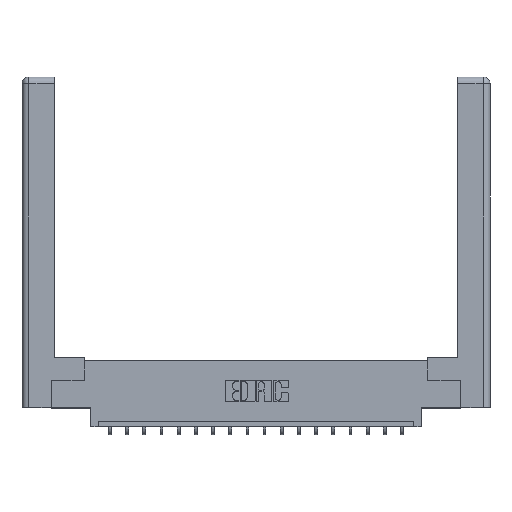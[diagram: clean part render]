
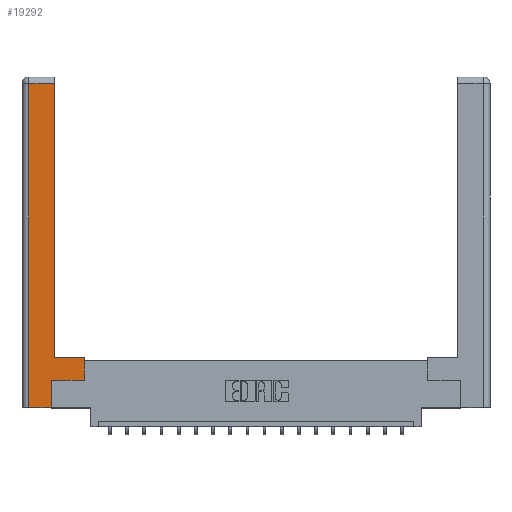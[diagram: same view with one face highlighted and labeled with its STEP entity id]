
A CAD part, top view. The second image highlights one B-rep face of the part: STEP entity #19292.
In plain terms, the highlighted planar face has unit normal (0, 0, 1).
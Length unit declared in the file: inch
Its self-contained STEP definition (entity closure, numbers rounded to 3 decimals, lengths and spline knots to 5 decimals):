
#159 = EDGE_CURVE ( 'NONE', #3786, #2519, #12593, .T. ) ;
#300 = EDGE_CURVE ( 'NONE', #6860, #7425, #4902, .T. ) ;
#514 = LINE ( 'NONE', #19225, #18014 ) ;
#951 = DIRECTION ( 'NONE',  ( -1., 0., 0. ) ) ;
#1025 = CARTESIAN_POINT ( 'NONE',  ( 0.565, 0.45, 0. ) ) ;
#1565 = CARTESIAN_POINT ( 'NONE',  ( 0.0615, 2.94, 0. ) ) ;
#1653 = ORIENTED_EDGE ( 'NONE', *, *, #16850, .T. ) ;
#1750 = ORIENTED_EDGE ( 'NONE', *, *, #300, .T. ) ;
#2519 = VERTEX_POINT ( 'NONE', #11934 ) ;
#2888 = DIRECTION ( 'NONE',  ( 0., 1., 0. ) ) ;
#2975 = DIRECTION ( 'NONE',  ( 1., 0., 0. ) ) ;
#3498 = CARTESIAN_POINT ( 'NONE',  ( 0.565, 0.245, 0. ) ) ;
#3678 = FACE_OUTER_BOUND ( 'NONE', #14730, .T. ) ;
#3786 = VERTEX_POINT ( 'NONE', #1025 ) ;
#3906 = CARTESIAN_POINT ( 'NONE',  ( 0., 0., 0. ) ) ;
#4070 = VERTEX_POINT ( 'NONE', #1565 ) ;
#4534 = CARTESIAN_POINT ( 'NONE',  ( 0.265, 0., 0. ) ) ;
#4902 = LINE ( 'NONE', #8746, #17951 ) ;
#5657 = DIRECTION ( 'NONE',  ( 0., 1., 0. ) ) ;
#5924 = ORIENTED_EDGE ( 'NONE', *, *, #6872, .T. ) ;
#6283 = LINE ( 'NONE', #10292, #14432 ) ;
#6556 = LINE ( 'NONE', #4534, #12621 ) ;
#6759 = ORIENTED_EDGE ( 'NONE', *, *, #8182, .T. ) ;
#6860 = VERTEX_POINT ( 'NONE', #7042 ) ;
#6872 = EDGE_CURVE ( 'NONE', #4070, #18617, #514, .T. ) ;
#7042 = CARTESIAN_POINT ( 'NONE',  ( 0.265, 0., 0. ) ) ;
#7152 = VECTOR ( 'NONE', #10842, 39.37008 ) ;
#7361 = DIRECTION ( 'NONE',  ( -1., 0., 0. ) ) ;
#7425 = VERTEX_POINT ( 'NONE', #11733 ) ;
#8073 = ORIENTED_EDGE ( 'NONE', *, *, #16611, .T. ) ;
#8082 = LINE ( 'NONE', #3498, #7152 ) ;
#8182 = EDGE_CURVE ( 'NONE', #19232, #4070, #11906, .T. ) ;
#8651 = VECTOR ( 'NONE', #11380, 39.37008 ) ;
#8746 = CARTESIAN_POINT ( 'NONE',  ( 0.265, 0.245, 0. ) ) ;
#10049 = EDGE_CURVE ( 'NONE', #2519, #19232, #15288, .T. ) ;
#10292 = CARTESIAN_POINT ( 'NONE',  ( 0.565, 0.45, 0. ) ) ;
#10531 = CARTESIAN_POINT ( 'NONE',  ( 0.0615, 2.94, 0. ) ) ;
#10842 = DIRECTION ( 'NONE',  ( 1., 0., 0. ) ) ;
#10862 = VECTOR ( 'NONE', #18126, 39.37008 ) ;
#10889 = ORIENTED_EDGE ( 'NONE', *, *, #10049, .T. ) ;
#11380 = DIRECTION ( 'NONE',  ( -1., 0., 0. ) ) ;
#11451 = DIRECTION ( 'NONE',  ( 0., 0., -1. ) ) ;
#11588 = EDGE_CURVE ( 'NONE', #7425, #14352, #8082, .T. ) ;
#11733 = CARTESIAN_POINT ( 'NONE',  ( 0.265, 0.245, 0. ) ) ;
#11906 = LINE ( 'NONE', #10531, #12377 ) ;
#11934 = CARTESIAN_POINT ( 'NONE',  ( 0.295, 0.45, 0. ) ) ;
#12377 = VECTOR ( 'NONE', #7361, 39.37008 ) ;
#12593 = LINE ( 'NONE', #18756, #8651 ) ;
#12621 = VECTOR ( 'NONE', #2975, 39.37008 ) ;
#13399 = ORIENTED_EDGE ( 'NONE', *, *, #159, .T. ) ;
#14352 = VERTEX_POINT ( 'NONE', #14885 ) ;
#14432 = VECTOR ( 'NONE', #2888, 39.37008 ) ;
#14730 = EDGE_LOOP ( 'NONE', ( #10889, #6759, #5924, #1653, #1750, #16818, #8073, #13399 ) ) ;
#14885 = CARTESIAN_POINT ( 'NONE',  ( 0.565, 0.245, 0. ) ) ;
#14909 = DIRECTION ( 'NONE',  ( 0., -1., 0. ) ) ;
#15288 = LINE ( 'NONE', #16642, #10862 ) ;
#16611 = EDGE_CURVE ( 'NONE', #14352, #3786, #6283, .T. ) ;
#16642 = CARTESIAN_POINT ( 'NONE',  ( 0.295, 3., 0. ) ) ;
#16729 = AXIS2_PLACEMENT_3D ( 'NONE', #3906, #11451, #951 ) ;
#16818 = ORIENTED_EDGE ( 'NONE', *, *, #11588, .T. ) ;
#16850 = EDGE_CURVE ( 'NONE', #18617, #6860, #6556, .T. ) ;
#17083 = CARTESIAN_POINT ( 'NONE',  ( 0.0615, 0., 0. ) ) ;
#17951 = VECTOR ( 'NONE', #5657, 39.37008 ) ;
#18014 = VECTOR ( 'NONE', #14909, 39.37008 ) ;
#18126 = DIRECTION ( 'NONE',  ( 0., 1., 0. ) ) ;
#18451 = CARTESIAN_POINT ( 'NONE',  ( 0.295, 2.94, 0. ) ) ;
#18617 = VERTEX_POINT ( 'NONE', #17083 ) ;
#18756 = CARTESIAN_POINT ( 'NONE',  ( 0.295, 0.45, 0. ) ) ;
#19025 = PLANE ( 'NONE',  #16729 ) ;
#19225 = CARTESIAN_POINT ( 'NONE',  ( 0.0615, 0., 0. ) ) ;
#19232 = VERTEX_POINT ( 'NONE', #18451 ) ;
#19292 = ADVANCED_FACE ( 'NONE', ( #3678 ), #19025, .F. ) ;
